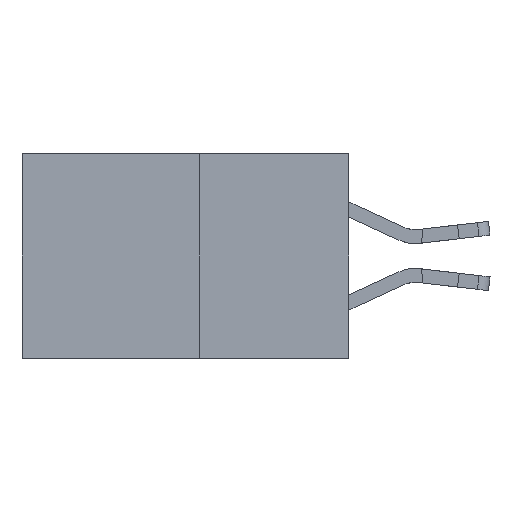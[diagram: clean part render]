
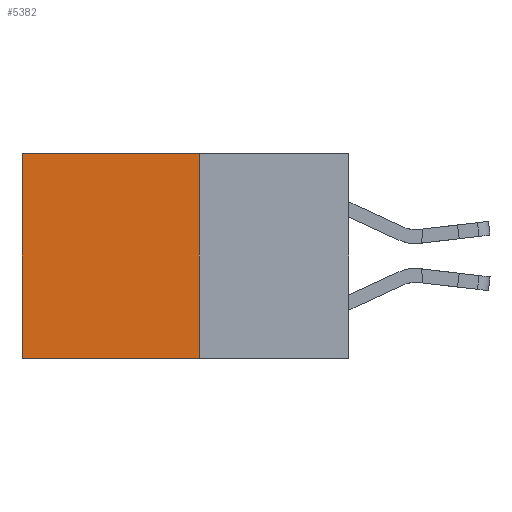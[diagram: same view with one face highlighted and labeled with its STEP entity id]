
A CAD part, left-side view. The second image highlights one B-rep face of the part: STEP entity #5382.
In plain terms, the highlighted planar face has unit normal (-1, 0, 0).
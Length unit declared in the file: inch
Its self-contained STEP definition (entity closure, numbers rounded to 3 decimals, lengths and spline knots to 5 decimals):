
#153 = AXIS2_PLACEMENT_3D ( 'NONE', #13670, #6490, #14820 ) ;
#592 = LINE ( 'NONE', #12172, #1407 ) ;
#1407 = VECTOR ( 'NONE', #4967, 39.37008 ) ;
#1957 = DIRECTION ( 'NONE',  ( 0., 0., -1. ) ) ;
#1993 = VECTOR ( 'NONE', #1957, 39.37008 ) ;
#2166 = ORIENTED_EDGE ( 'NONE', *, *, #5826, .T. ) ;
#2324 = LINE ( 'NONE', #6363, #14662 ) ;
#2814 = CARTESIAN_POINT ( 'NONE',  ( 0.277, 0.59, 0. ) ) ;
#4020 = ORIENTED_EDGE ( 'NONE', *, *, #13591, .T. ) ;
#4967 = DIRECTION ( 'NONE',  ( 0., 0., -1. ) ) ;
#5132 = ORIENTED_EDGE ( 'NONE', *, *, #11011, .F. ) ;
#5290 = PLANE ( 'NONE',  #153 ) ;
#5382 = ADVANCED_FACE ( 'NONE', ( #10650 ), #5290, .F. ) ;
#5522 = EDGE_CURVE ( 'NONE', #15361, #6464, #11620, .T. ) ;
#5528 = CARTESIAN_POINT ( 'NONE',  ( 0.277, 0.27, 0. ) ) ;
#5531 = CARTESIAN_POINT ( 'NONE',  ( 0.277, 0.27, -0.37 ) ) ;
#5826 = EDGE_CURVE ( 'NONE', #13620, #11742, #592, .T. ) ;
#6363 = CARTESIAN_POINT ( 'NONE',  ( 0.277, 0.27, 0. ) ) ;
#6464 = VERTEX_POINT ( 'NONE', #14637 ) ;
#6490 = DIRECTION ( 'NONE',  ( 1., 0., 0. ) ) ;
#6789 = CARTESIAN_POINT ( 'NONE',  ( 0.277, 0.27, -0.37 ) ) ;
#8554 = LINE ( 'NONE', #6789, #14156 ) ;
#9196 = DIRECTION ( 'NONE',  ( 0., 1., 0. ) ) ;
#10650 = FACE_OUTER_BOUND ( 'NONE', #10979, .T. ) ;
#10979 = EDGE_LOOP ( 'NONE', ( #2166, #5132, #13220, #4020 ) ) ;
#11011 = EDGE_CURVE ( 'NONE', #6464, #11742, #8554, .T. ) ;
#11620 = LINE ( 'NONE', #5531, #1993 ) ;
#11742 = VERTEX_POINT ( 'NONE', #13849 ) ;
#12172 = CARTESIAN_POINT ( 'NONE',  ( 0.277, 0.59, -0.37 ) ) ;
#13220 = ORIENTED_EDGE ( 'NONE', *, *, #5522, .F. ) ;
#13552 = DIRECTION ( 'NONE',  ( 0., 1., 0. ) ) ;
#13591 = EDGE_CURVE ( 'NONE', #15361, #13620, #2324, .T. ) ;
#13620 = VERTEX_POINT ( 'NONE', #2814 ) ;
#13670 = CARTESIAN_POINT ( 'NONE',  ( 0.277, 0.27, -0.37 ) ) ;
#13849 = CARTESIAN_POINT ( 'NONE',  ( 0.277, 0.59, -0.37 ) ) ;
#14156 = VECTOR ( 'NONE', #9196, 39.37008 ) ;
#14637 = CARTESIAN_POINT ( 'NONE',  ( 0.277, 0.27, -0.37 ) ) ;
#14662 = VECTOR ( 'NONE', #13552, 39.37008 ) ;
#14820 = DIRECTION ( 'NONE',  ( 0., 0., -1. ) ) ;
#15361 = VERTEX_POINT ( 'NONE', #5528 ) ;
